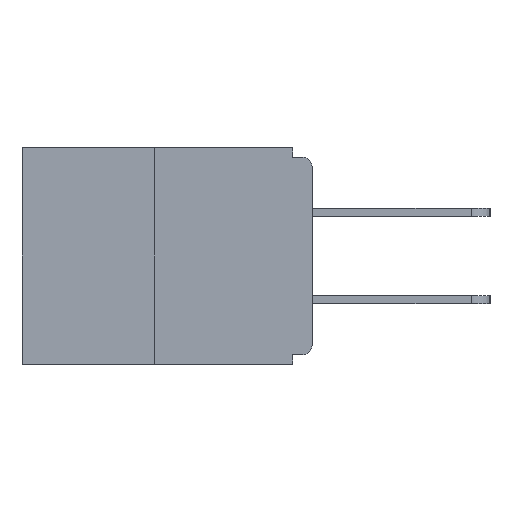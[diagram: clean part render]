
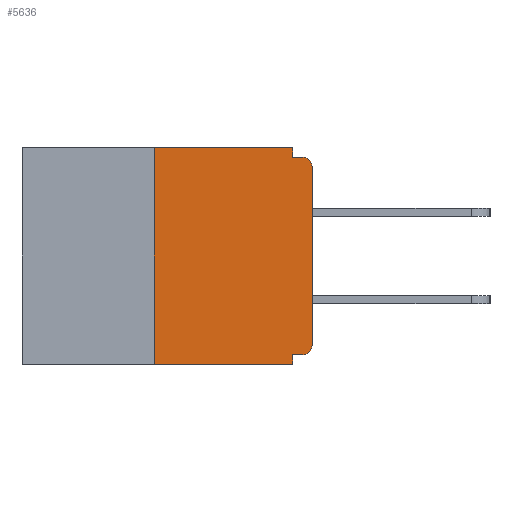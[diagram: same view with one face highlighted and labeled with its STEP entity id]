
A CAD part, left-side view. The second image highlights one B-rep face of the part: STEP entity #5636.
In plain terms, the highlighted planar face has unit normal (-1, 0, 0).
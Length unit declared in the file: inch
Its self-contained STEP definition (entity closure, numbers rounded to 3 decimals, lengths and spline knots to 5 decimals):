
#433 = EDGE_CURVE ( 'NONE', #15703, #11830, #18036, .T. ) ;
#979 = ORIENTED_EDGE ( 'NONE', *, *, #9455, .F. ) ;
#1223 = LINE ( 'NONE', #15662, #15947 ) ;
#1278 = AXIS2_PLACEMENT_3D ( 'NONE', #7531, #5827, #18346 ) ;
#1288 = VERTEX_POINT ( 'NONE', #12413 ) ;
#1422 = VERTEX_POINT ( 'NONE', #6605 ) ;
#1516 = CARTESIAN_POINT ( 'NONE',  ( 0., 0., -0.328 ) ) ;
#1704 = VECTOR ( 'NONE', #1841, 39.37008 ) ;
#1732 = DIRECTION ( 'NONE',  ( 0., 0., -1. ) ) ;
#1841 = DIRECTION ( 'NONE',  ( 0., -1., 0. ) ) ;
#1898 = LINE ( 'NONE', #6447, #13463 ) ;
#2646 = VERTEX_POINT ( 'NONE', #13571 ) ;
#2689 = ORIENTED_EDGE ( 'NONE', *, *, #16890, .F. ) ;
#3157 = ORIENTED_EDGE ( 'NONE', *, *, #12673, .T. ) ;
#3267 = VERTEX_POINT ( 'NONE', #5545 ) ;
#3483 = ORIENTED_EDGE ( 'NONE', *, *, #6486, .F. ) ;
#4063 = ORIENTED_EDGE ( 'NONE', *, *, #11454, .T. ) ;
#4315 = AXIS2_PLACEMENT_3D ( 'NONE', #6468, #12475, #4863 ) ;
#4731 = CARTESIAN_POINT ( 'NONE',  ( 0., 0., -0.015 ) ) ;
#4822 = CARTESIAN_POINT ( 'NONE',  ( 0., 0.031, 0. ) ) ;
#4863 = DIRECTION ( 'NONE',  ( 0., 0., -1. ) ) ;
#5545 = CARTESIAN_POINT ( 'NONE',  ( 0., 0.031, -0.343 ) ) ;
#5636 = ADVANCED_FACE ( 'NONE', ( #10688 ), #17704, .F. ) ;
#5787 = AXIS2_PLACEMENT_3D ( 'NONE', #19276, #8851, #19604 ) ;
#5827 = DIRECTION ( 'NONE',  ( -1., 0., 0. ) ) ;
#6024 = EDGE_CURVE ( 'NONE', #8252, #1422, #13248, .T. ) ;
#6098 = CARTESIAN_POINT ( 'NONE',  ( 0., 0.46, 0. ) ) ;
#6447 = CARTESIAN_POINT ( 'NONE',  ( 0., 0.031, -0.343 ) ) ;
#6468 = CARTESIAN_POINT ( 'NONE',  ( 0., 0.015, -0.313 ) ) ;
#6486 = EDGE_CURVE ( 'NONE', #1288, #15703, #19054, .T. ) ;
#6600 = CIRCLE ( 'NONE', #4315, 0.015 ) ;
#6605 = CARTESIAN_POINT ( 'NONE',  ( 0., 0., -0.03 ) ) ;
#7205 = VECTOR ( 'NONE', #7564, 39.37008 ) ;
#7497 = ORIENTED_EDGE ( 'NONE', *, *, #17352, .T. ) ;
#7531 = CARTESIAN_POINT ( 'NONE',  ( 0., 0.015, -0.03 ) ) ;
#7564 = DIRECTION ( 'NONE',  ( 0., 1., 0. ) ) ;
#8044 = EDGE_LOOP ( 'NONE', ( #3483, #2689, #3157, #15125, #979, #4063, #8255, #7497, #17310, #19944 ) ) ;
#8252 = VERTEX_POINT ( 'NONE', #13714 ) ;
#8255 = ORIENTED_EDGE ( 'NONE', *, *, #6024, .T. ) ;
#8430 = CARTESIAN_POINT ( 'NONE',  ( 0., 0.25, -0.343 ) ) ;
#8458 = VECTOR ( 'NONE', #1732, 39.37008 ) ;
#8851 = DIRECTION ( 'NONE',  ( 1., 0., 0. ) ) ;
#9455 = EDGE_CURVE ( 'NONE', #18952, #18205, #19509, .T. ) ;
#10108 = EDGE_CURVE ( 'NONE', #11830, #2646, #16491, .T. ) ;
#10688 = FACE_OUTER_BOUND ( 'NONE', #8044, .T. ) ;
#11177 = DIRECTION ( 'NONE',  ( 0., 0., -1. ) ) ;
#11202 = CARTESIAN_POINT ( 'NONE',  ( 0., 0.46, -0.343 ) ) ;
#11454 = EDGE_CURVE ( 'NONE', #18952, #8252, #6600, .T. ) ;
#11594 = DIRECTION ( 'NONE',  ( 0., 0., 1. ) ) ;
#11745 = CARTESIAN_POINT ( 'NONE',  ( 0., 0.015, -0.328 ) ) ;
#11830 = VERTEX_POINT ( 'NONE', #12330 ) ;
#12330 = CARTESIAN_POINT ( 'NONE',  ( 0., 0.031, -0.015 ) ) ;
#12356 = LINE ( 'NONE', #11202, #1704 ) ;
#12413 = CARTESIAN_POINT ( 'NONE',  ( 0., 0.25, 0. ) ) ;
#12475 = DIRECTION ( 'NONE',  ( -1., 0., 0. ) ) ;
#12673 = EDGE_CURVE ( 'NONE', #19489, #3267, #12356, .T. ) ;
#12897 = CARTESIAN_POINT ( 'NONE',  ( 0., 0.031, -0.328 ) ) ;
#13033 = VECTOR ( 'NONE', #15160, 39.37008 ) ;
#13248 = LINE ( 'NONE', #17669, #18325 ) ;
#13463 = VECTOR ( 'NONE', #11177, 39.37008 ) ;
#13571 = CARTESIAN_POINT ( 'NONE',  ( 0., 0.015, -0.015 ) ) ;
#13677 = EDGE_CURVE ( 'NONE', #18205, #3267, #1898, .T. ) ;
#13714 = CARTESIAN_POINT ( 'NONE',  ( 0., 0., -0.313 ) ) ;
#15125 = ORIENTED_EDGE ( 'NONE', *, *, #13677, .F. ) ;
#15160 = DIRECTION ( 'NONE',  ( 0., -1., 0. ) ) ;
#15662 = CARTESIAN_POINT ( 'NONE',  ( 0., 0.25, 0. ) ) ;
#15703 = VERTEX_POINT ( 'NONE', #15996 ) ;
#15947 = VECTOR ( 'NONE', #18840, 39.37008 ) ;
#15996 = CARTESIAN_POINT ( 'NONE',  ( 0., 0.031, 0. ) ) ;
#16491 = LINE ( 'NONE', #4731, #19911 ) ;
#16808 = DIRECTION ( 'NONE',  ( 0., -1., 0. ) ) ;
#16890 = EDGE_CURVE ( 'NONE', #19489, #1288, #1223, .T. ) ;
#17310 = ORIENTED_EDGE ( 'NONE', *, *, #10108, .F. ) ;
#17352 = EDGE_CURVE ( 'NONE', #1422, #2646, #18842, .T. ) ;
#17669 = CARTESIAN_POINT ( 'NONE',  ( 0., 0., 0. ) ) ;
#17704 = PLANE ( 'NONE',  #5787 ) ;
#18036 = LINE ( 'NONE', #4822, #8458 ) ;
#18205 = VERTEX_POINT ( 'NONE', #12897 ) ;
#18325 = VECTOR ( 'NONE', #11594, 39.37008 ) ;
#18346 = DIRECTION ( 'NONE',  ( 0., 0., -1. ) ) ;
#18840 = DIRECTION ( 'NONE',  ( 0., 0., 1. ) ) ;
#18842 = CIRCLE ( 'NONE', #1278, 0.015 ) ;
#18952 = VERTEX_POINT ( 'NONE', #11745 ) ;
#19054 = LINE ( 'NONE', #6098, #13033 ) ;
#19276 = CARTESIAN_POINT ( 'NONE',  ( 0., 0.46, 0. ) ) ;
#19489 = VERTEX_POINT ( 'NONE', #8430 ) ;
#19509 = LINE ( 'NONE', #1516, #7205 ) ;
#19604 = DIRECTION ( 'NONE',  ( 0., 0., -1. ) ) ;
#19911 = VECTOR ( 'NONE', #16808, 39.37008 ) ;
#19944 = ORIENTED_EDGE ( 'NONE', *, *, #433, .F. ) ;
